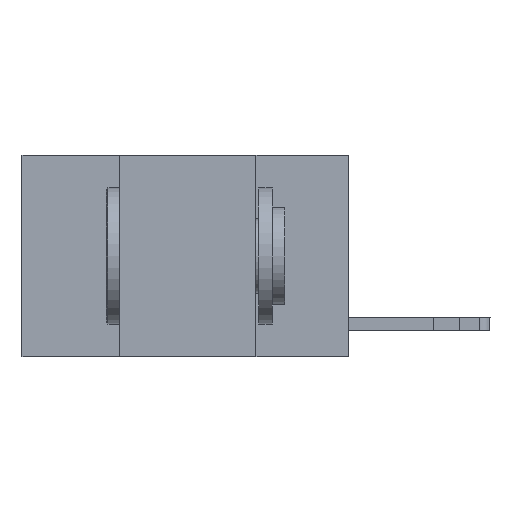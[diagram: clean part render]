
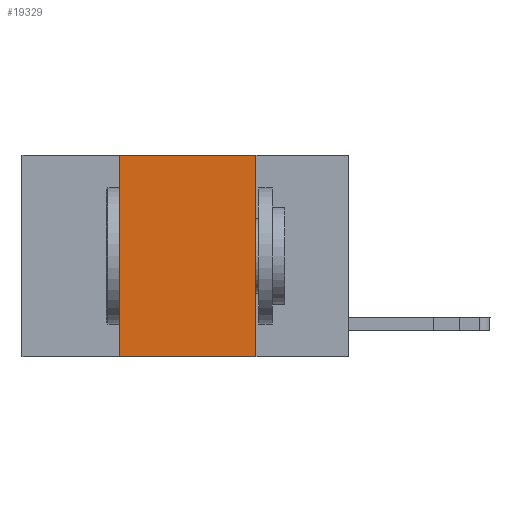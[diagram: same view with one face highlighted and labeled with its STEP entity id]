
A CAD part, left-side view. The second image highlights one B-rep face of the part: STEP entity #19329.
In plain terms, the highlighted planar face has unit normal (-1, 0, 0).
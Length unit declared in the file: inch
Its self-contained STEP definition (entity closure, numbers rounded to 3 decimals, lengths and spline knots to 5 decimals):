
#1366 = ORIENTED_EDGE ( 'NONE', *, *, #17105, .F. ) ;
#1429 = DIRECTION ( 'NONE',  ( 0., 0., -1. ) ) ;
#1556 = VECTOR ( 'NONE', #12062, 39.37008 ) ;
#3344 = VECTOR ( 'NONE', #1429, 39.37008 ) ;
#4669 = LINE ( 'NONE', #18459, #3344 ) ;
#4744 = DIRECTION ( 'NONE',  ( 1., 0., 0. ) ) ;
#4897 = LINE ( 'NONE', #11042, #5872 ) ;
#5749 = VECTOR ( 'NONE', #18322, 39.37008 ) ;
#5872 = VECTOR ( 'NONE', #7836, 39.37008 ) ;
#6066 = LINE ( 'NONE', #16725, #5749 ) ;
#6854 = AXIS2_PLACEMENT_3D ( 'NONE', #18247, #4744, #18441 ) ;
#7606 = EDGE_CURVE ( 'NONE', #13622, #11542, #4669, .T. ) ;
#7836 = DIRECTION ( 'NONE',  ( 0., -1., 0. ) ) ;
#8133 = ORIENTED_EDGE ( 'NONE', *, *, #8413, .T. ) ;
#8413 = EDGE_CURVE ( 'NONE', #16404, #11542, #6066, .T. ) ;
#8461 = CARTESIAN_POINT ( 'NONE',  ( 0., 0.42, 0. ) ) ;
#8729 = ORIENTED_EDGE ( 'NONE', *, *, #7606, .F. ) ;
#8925 = LINE ( 'NONE', #11861, #1556 ) ;
#9490 = FACE_OUTER_BOUND ( 'NONE', #15025, .T. ) ;
#9977 = CARTESIAN_POINT ( 'NONE',  ( 0., 0.17, -0.37 ) ) ;
#11042 = CARTESIAN_POINT ( 'NONE',  ( 0., 0.6, 0. ) ) ;
#11325 = ORIENTED_EDGE ( 'NONE', *, *, #12772, .F. ) ;
#11542 = VERTEX_POINT ( 'NONE', #9977 ) ;
#11861 = CARTESIAN_POINT ( 'NONE',  ( 0., 0.42, 0. ) ) ;
#11989 = CARTESIAN_POINT ( 'NONE',  ( 0., 0.17, 0. ) ) ;
#12062 = DIRECTION ( 'NONE',  ( 0., 0., 1. ) ) ;
#12405 = PLANE ( 'NONE',  #6854 ) ;
#12772 = EDGE_CURVE ( 'NONE', #16404, #16205, #8925, .T. ) ;
#13622 = VERTEX_POINT ( 'NONE', #11989 ) ;
#14131 = CARTESIAN_POINT ( 'NONE',  ( 0., 0.42, -0.37 ) ) ;
#15025 = EDGE_LOOP ( 'NONE', ( #8729, #1366, #11325, #8133 ) ) ;
#16205 = VERTEX_POINT ( 'NONE', #8461 ) ;
#16404 = VERTEX_POINT ( 'NONE', #14131 ) ;
#16725 = CARTESIAN_POINT ( 'NONE',  ( 0., 0.6, -0.37 ) ) ;
#17105 = EDGE_CURVE ( 'NONE', #16205, #13622, #4897, .T. ) ;
#18247 = CARTESIAN_POINT ( 'NONE',  ( 0., 0.6, 0. ) ) ;
#18322 = DIRECTION ( 'NONE',  ( 0., -1., 0. ) ) ;
#18441 = DIRECTION ( 'NONE',  ( 0., 0., -1. ) ) ;
#18459 = CARTESIAN_POINT ( 'NONE',  ( 0., 0.17, 0. ) ) ;
#19329 = ADVANCED_FACE ( 'NONE', ( #9490 ), #12405, .F. ) ;
